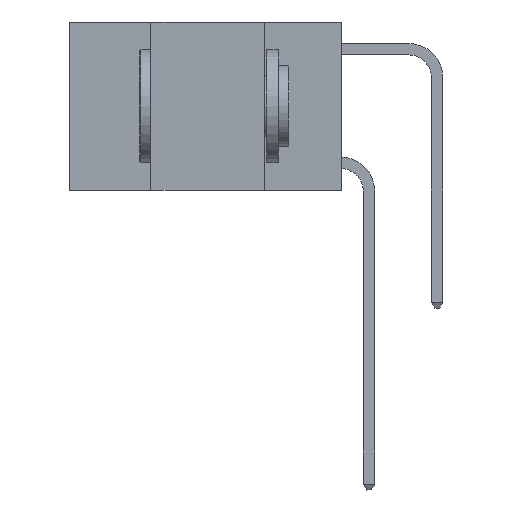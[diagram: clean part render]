
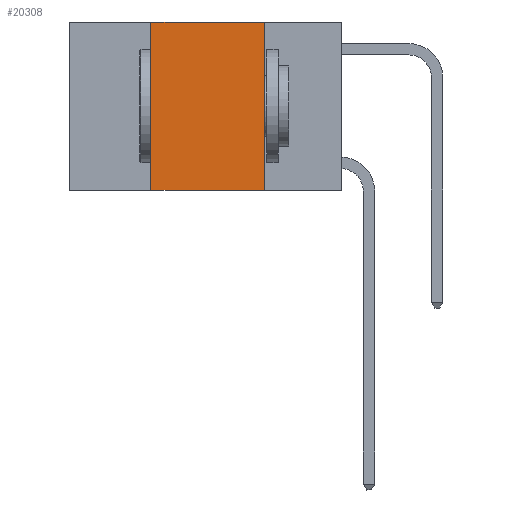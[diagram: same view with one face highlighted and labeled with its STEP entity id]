
A CAD part, left-side view. The second image highlights one B-rep face of the part: STEP entity #20308.
In plain terms, the highlighted planar face has unit normal (-1, 0, 0).
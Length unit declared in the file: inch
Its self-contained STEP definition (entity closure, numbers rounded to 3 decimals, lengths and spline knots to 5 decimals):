
#256 = AXIS2_PLACEMENT_3D ( 'NONE', #23365, #9013, #25799 ) ;
#2156 = VERTEX_POINT ( 'NONE', #9536 ) ;
#2560 = CARTESIAN_POINT ( 'NONE',  ( 0., 0.6, 0. ) ) ;
#2703 = CARTESIAN_POINT ( 'NONE',  ( 0., 0.6, -0.37 ) ) ;
#2953 = EDGE_CURVE ( 'NONE', #18028, #15447, #14135, .T. ) ;
#3050 = ORIENTED_EDGE ( 'NONE', *, *, #11045, .F. ) ;
#3805 = ORIENTED_EDGE ( 'NONE', *, *, #24991, .T. ) ;
#4148 = PLANE ( 'NONE',  #256 ) ;
#5115 = DIRECTION ( 'NONE',  ( 0., -1., 0. ) ) ;
#7038 = LINE ( 'NONE', #9074, #19039 ) ;
#8002 = EDGE_LOOP ( 'NONE', ( #8710, #3050, #28604, #3805 ) ) ;
#8227 = LINE ( 'NONE', #2703, #26617 ) ;
#8368 = VECTOR ( 'NONE', #24201, 39.37008 ) ;
#8710 = ORIENTED_EDGE ( 'NONE', *, *, #26180, .F. ) ;
#9013 = DIRECTION ( 'NONE',  ( 1., 0., 0. ) ) ;
#9074 = CARTESIAN_POINT ( 'NONE',  ( 0., 0.17, 0. ) ) ;
#9105 = FACE_OUTER_BOUND ( 'NONE', #8002, .T. ) ;
#9209 = CARTESIAN_POINT ( 'NONE',  ( 0., 0.17, 0. ) ) ;
#9536 = CARTESIAN_POINT ( 'NONE',  ( 0., 0.17, -0.37 ) ) ;
#10893 = VERTEX_POINT ( 'NONE', #9209 ) ;
#11045 = EDGE_CURVE ( 'NONE', #15447, #10893, #14773, .T. ) ;
#13930 = DIRECTION ( 'NONE',  ( 0., 0., -1. ) ) ;
#14135 = LINE ( 'NONE', #14383, #26858 ) ;
#14383 = CARTESIAN_POINT ( 'NONE',  ( 0., 0.42, 0. ) ) ;
#14773 = LINE ( 'NONE', #2560, #8368 ) ;
#15447 = VERTEX_POINT ( 'NONE', #23514 ) ;
#18028 = VERTEX_POINT ( 'NONE', #30599 ) ;
#19039 = VECTOR ( 'NONE', #13930, 39.37008 ) ;
#20308 = ADVANCED_FACE ( 'NONE', ( #9105 ), #4148, .F. ) ;
#23365 = CARTESIAN_POINT ( 'NONE',  ( 0., 0.6, 0. ) ) ;
#23514 = CARTESIAN_POINT ( 'NONE',  ( 0., 0.42, 0. ) ) ;
#24201 = DIRECTION ( 'NONE',  ( 0., -1., 0. ) ) ;
#24991 = EDGE_CURVE ( 'NONE', #18028, #2156, #8227, .T. ) ;
#25799 = DIRECTION ( 'NONE',  ( 0., 0., -1. ) ) ;
#26180 = EDGE_CURVE ( 'NONE', #10893, #2156, #7038, .T. ) ;
#26617 = VECTOR ( 'NONE', #5115, 39.37008 ) ;
#26858 = VECTOR ( 'NONE', #28727, 39.37008 ) ;
#28604 = ORIENTED_EDGE ( 'NONE', *, *, #2953, .F. ) ;
#28727 = DIRECTION ( 'NONE',  ( 0., 0., 1. ) ) ;
#30599 = CARTESIAN_POINT ( 'NONE',  ( 0., 0.42, -0.37 ) ) ;
